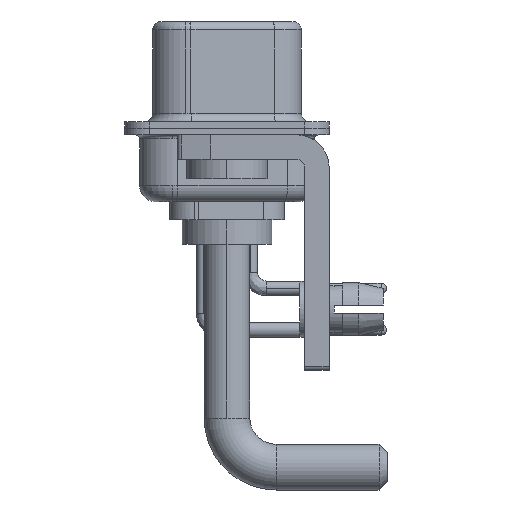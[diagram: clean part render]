
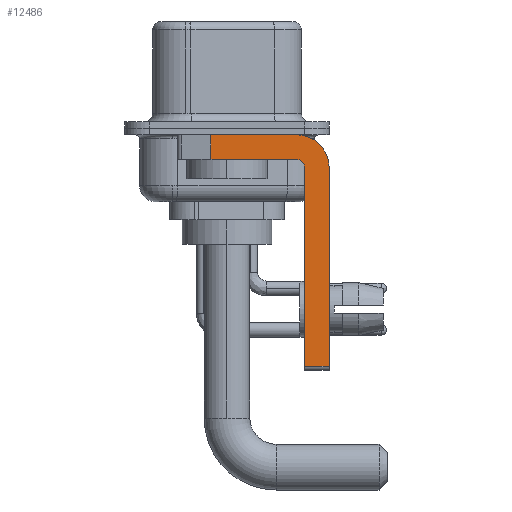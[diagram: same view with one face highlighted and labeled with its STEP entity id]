
A CAD part, left-side view. The second image highlights one B-rep face of the part: STEP entity #12486.
In plain terms, the highlighted planar face has unit normal (-1, 0, 0).
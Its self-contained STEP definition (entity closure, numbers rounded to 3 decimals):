
#95 = VERTEX_POINT ( 'NONE', #27566 ) ;
#152 = ORIENTED_EDGE ( 'NONE', *, *, #5260, .T. ) ;
#467 = CARTESIAN_POINT ( 'NONE',  ( -2.9, 3., -0.4 ) ) ;
#614 = ORIENTED_EDGE ( 'NONE', *, *, #20353, .T. ) ;
#1548 = CARTESIAN_POINT ( 'NONE',  ( -2.9, 0.978, -1.9 ) ) ;
#2015 = CARTESIAN_POINT ( 'NONE',  ( -2.9, -4.25, -2.4 ) ) ;
#3087 = LINE ( 'NONE', #11796, #17660 ) ;
#3311 = CARTESIAN_POINT ( 'NONE',  ( -2.9, -6.25, -14.55 ) ) ;
#3544 = ORIENTED_EDGE ( 'NONE', *, *, #5129, .F. ) ;
#3765 = VERTEX_POINT ( 'NONE', #16418 ) ;
#3988 = VERTEX_POINT ( 'NONE', #4962 ) ;
#4369 = CARTESIAN_POINT ( 'NONE',  ( -2.9, -6.25, -2.4 ) ) ;
#4677 = PLANE ( 'NONE',  #18857 ) ;
#4962 = CARTESIAN_POINT ( 'NONE',  ( -2.9, -4.75, -2.4 ) ) ;
#5129 = EDGE_CURVE ( 'NONE', #95, #16183, #11923, .T. ) ;
#5260 = EDGE_CURVE ( 'NONE', #9450, #16183, #26032, .T. ) ;
#6551 = CARTESIAN_POINT ( 'NONE',  ( -2.9, -4.25, -2.4 ) ) ;
#6777 = EDGE_CURVE ( 'NONE', #14232, #8990, #3087, .T. ) ;
#6823 = EDGE_LOOP ( 'NONE', ( #9198, #152, #3544, #21817, #23861, #614, #23264, #16066 ) ) ;
#7103 = DIRECTION ( 'NONE',  ( 0., 0., -1. ) ) ;
#7713 = AXIS2_PLACEMENT_3D ( 'NONE', #9434, #18558, #27239 ) ;
#8609 = LINE ( 'NONE', #25988, #13657 ) ;
#8861 = EDGE_CURVE ( 'NONE', #9450, #3765, #15878, .T. ) ;
#8990 = VERTEX_POINT ( 'NONE', #3311 ) ;
#9113 = EDGE_CURVE ( 'NONE', #25640, #3988, #8609, .T. ) ;
#9198 = ORIENTED_EDGE ( 'NONE', *, *, #8861, .F. ) ;
#9434 = CARTESIAN_POINT ( 'NONE',  ( -2.9, -4.25, -2.4 ) ) ;
#9448 = AXIS2_PLACEMENT_3D ( 'NONE', #2015, #10734, #21275 ) ;
#9450 = VERTEX_POINT ( 'NONE', #15843 ) ;
#9468 = EDGE_CURVE ( 'NONE', #3765, #14232, #19993, .T. ) ;
#10093 = CARTESIAN_POINT ( 'NONE',  ( -2.9, -4.25, -1.9 ) ) ;
#10734 = DIRECTION ( 'NONE',  ( -1., 0., 0. ) ) ;
#11796 = CARTESIAN_POINT ( 'NONE',  ( -2.9, -6.25, -2.4 ) ) ;
#11923 = LINE ( 'NONE', #10093, #16211 ) ;
#12358 = DIRECTION ( 'NONE',  ( 0., 1., 0. ) ) ;
#12486 = ADVANCED_FACE ( 'NONE', ( #15522 ), #4677, .F. ) ;
#13330 = CARTESIAN_POINT ( 'NONE',  ( -2.9, -4.75, -14.55 ) ) ;
#13371 = DIRECTION ( 'NONE',  ( 1., 0., 0. ) ) ;
#13657 = VECTOR ( 'NONE', #16875, 1000. ) ;
#14127 = VECTOR ( 'NONE', #24015, 1000. ) ;
#14232 = VERTEX_POINT ( 'NONE', #4369 ) ;
#15522 = FACE_OUTER_BOUND ( 'NONE', #6823, .T. ) ;
#15843 = CARTESIAN_POINT ( 'NONE',  ( -2.9, 0.978, -0.4 ) ) ;
#15878 = LINE ( 'NONE', #467, #14127 ) ;
#16066 = ORIENTED_EDGE ( 'NONE', *, *, #9468, .F. ) ;
#16183 = VERTEX_POINT ( 'NONE', #1548 ) ;
#16211 = VECTOR ( 'NONE', #12358, 1000. ) ;
#16418 = CARTESIAN_POINT ( 'NONE',  ( -2.9, -4.25, -0.4 ) ) ;
#16742 = CARTESIAN_POINT ( 'NONE',  ( -2.9, -4.25, -14.55 ) ) ;
#16875 = DIRECTION ( 'NONE',  ( 0., 0., 1. ) ) ;
#17210 = DIRECTION ( 'NONE',  ( 0., 0., -1. ) ) ;
#17660 = VECTOR ( 'NONE', #20492, 1000. ) ;
#18558 = DIRECTION ( 'NONE',  ( 1., 0., 0. ) ) ;
#18744 = DIRECTION ( 'NONE',  ( 0., -1., 0. ) ) ;
#18857 = AXIS2_PLACEMENT_3D ( 'NONE', #6551, #13371, #7103 ) ;
#19614 = CARTESIAN_POINT ( 'NONE',  ( -2.9, 0.978, -1.9 ) ) ;
#19993 = CIRCLE ( 'NONE', #7713, 2. ) ;
#20353 = EDGE_CURVE ( 'NONE', #25640, #8990, #21003, .T. ) ;
#20492 = DIRECTION ( 'NONE',  ( 0., 0., -1. ) ) ;
#21003 = LINE ( 'NONE', #16742, #23159 ) ;
#21275 = DIRECTION ( 'NONE',  ( 0., 0., 1. ) ) ;
#21731 = CIRCLE ( 'NONE', #9448, 0.5 ) ;
#21817 = ORIENTED_EDGE ( 'NONE', *, *, #26386, .F. ) ;
#23047 = VECTOR ( 'NONE', #17210, 1000. ) ;
#23159 = VECTOR ( 'NONE', #18744, 1000. ) ;
#23264 = ORIENTED_EDGE ( 'NONE', *, *, #6777, .F. ) ;
#23861 = ORIENTED_EDGE ( 'NONE', *, *, #9113, .F. ) ;
#24015 = DIRECTION ( 'NONE',  ( 0., -1., 0. ) ) ;
#25640 = VERTEX_POINT ( 'NONE', #13330 ) ;
#25988 = CARTESIAN_POINT ( 'NONE',  ( -2.9, -4.75, -14.8 ) ) ;
#26032 = LINE ( 'NONE', #19614, #23047 ) ;
#26386 = EDGE_CURVE ( 'NONE', #3988, #95, #21731, .T. ) ;
#27239 = DIRECTION ( 'NONE',  ( 0., 0., -1. ) ) ;
#27566 = CARTESIAN_POINT ( 'NONE',  ( -2.9, -4.25, -1.9 ) ) ;
